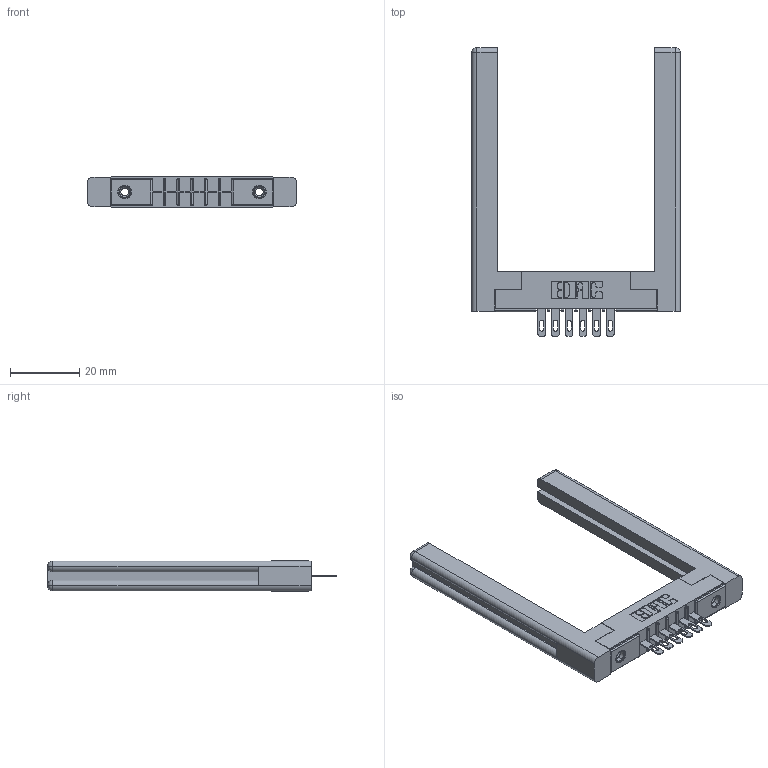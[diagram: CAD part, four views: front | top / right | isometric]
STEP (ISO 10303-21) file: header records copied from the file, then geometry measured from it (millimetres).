
FILE_DESCRIPTION (( 'STEP AP203' ), '1' );
FILE_NAME ('356-006-500-158.STEP', '2018-07-31T06:11:24', ( '' ), ( '' ), 'SwSTEP 2.0', 'SolidWorks 2016', '' );
FILE_SCHEMA (( 'CONFIG_CONTROL_DESIGN' ));
Length unit declared in the file: inch
Products named in the file (5): 306 Part_.156 Dia; 306-290-001_100; 345-250-001_345-250-001-102; 307-220-058; 356-006-500-158
Assembly tree (11 placements, depth 2):
  356-006-500-158
    306 Part_.156 Dia
    306-290-001_100  x6
    345-250-001_345-250-001-102  x2
    307-220-058  x2
Bounding box: 60.4 x 83.52 x 8.71 mm (x, y, z)
Volume: 11721.7 mm3; surface area: 10917.3 mm2
Topology: 11 solids, 11 shells, 714 faces, 1960 edges, 1260 vertices
Faces by surface type: plane 452, cylinder 214, sphere 24, cone 12, torus 12
Entity records: 13056 total; most frequent: CARTESIAN_POINT 2196, DIRECTION 2125, ORIENTED_EDGE 2114, EDGE_CURVE 1057, LINE 799, VECTOR 799, VERTEX_POINT 680, AXIS2_PLACEMENT_3D 663
